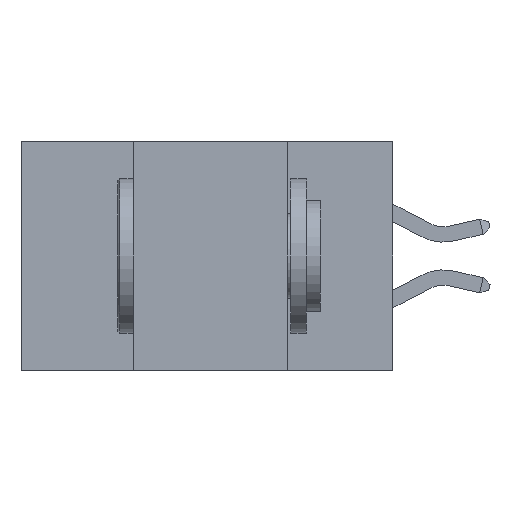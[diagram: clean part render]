
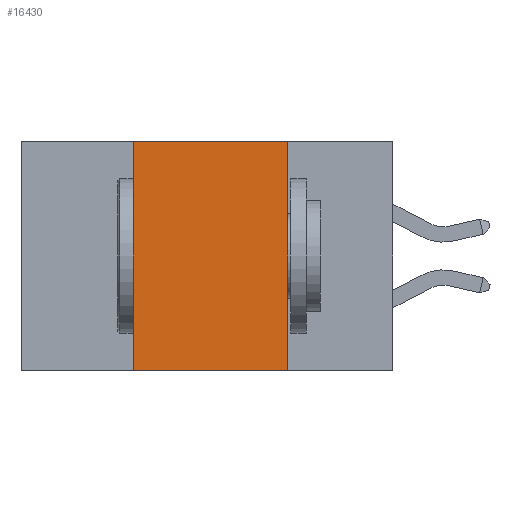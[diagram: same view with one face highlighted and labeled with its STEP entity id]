
A CAD part, left-side view. The second image highlights one B-rep face of the part: STEP entity #16430.
In plain terms, the highlighted planar face has unit normal (-1, 0, 0).
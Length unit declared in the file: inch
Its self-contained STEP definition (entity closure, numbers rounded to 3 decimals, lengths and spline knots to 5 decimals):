
#377 = VERTEX_POINT ( 'NONE', #13015 ) ;
#747 = VECTOR ( 'NONE', #12269, 39.37008 ) ;
#751 = EDGE_CURVE ( 'NONE', #3571, #23676, #10433, .T. ) ;
#1999 = FACE_OUTER_BOUND ( 'NONE', #18208, .T. ) ;
#2033 = CARTESIAN_POINT ( 'NONE',  ( 0., 0.17, 0. ) ) ;
#3480 = CARTESIAN_POINT ( 'NONE',  ( 0., 0.42, 0. ) ) ;
#3571 = VERTEX_POINT ( 'NONE', #21152 ) ;
#5234 = LINE ( 'NONE', #22747, #747 ) ;
#5465 = EDGE_CURVE ( 'NONE', #15761, #377, #5234, .T. ) ;
#5476 = PLANE ( 'NONE',  #8783 ) ;
#5738 = LINE ( 'NONE', #25685, #24884 ) ;
#5757 = DIRECTION ( 'NONE',  ( 0., 0., 1. ) ) ;
#6698 = LINE ( 'NONE', #3480, #24538 ) ;
#7764 = CARTESIAN_POINT ( 'NONE',  ( 0., 0.6, 0. ) ) ;
#8783 = AXIS2_PLACEMENT_3D ( 'NONE', #7764, #26142, #13625 ) ;
#10433 = LINE ( 'NONE', #17505, #19485 ) ;
#11803 = ORIENTED_EDGE ( 'NONE', *, *, #5465, .T. ) ;
#12073 = ORIENTED_EDGE ( 'NONE', *, *, #18575, .F. ) ;
#12269 = DIRECTION ( 'NONE',  ( 0., -1., 0. ) ) ;
#13015 = CARTESIAN_POINT ( 'NONE',  ( 0., 0.17, -0.37 ) ) ;
#13625 = DIRECTION ( 'NONE',  ( 0., 0., -1. ) ) ;
#13875 = ORIENTED_EDGE ( 'NONE', *, *, #18766, .F. ) ;
#15761 = VERTEX_POINT ( 'NONE', #23982 ) ;
#16430 = ADVANCED_FACE ( 'NONE', ( #1999 ), #5476, .F. ) ;
#17505 = CARTESIAN_POINT ( 'NONE',  ( 0., 0.6, 0. ) ) ;
#17787 = DIRECTION ( 'NONE',  ( 0., 0., -1. ) ) ;
#18208 = EDGE_LOOP ( 'NONE', ( #12073, #26581, #13875, #11803 ) ) ;
#18575 = EDGE_CURVE ( 'NONE', #23676, #377, #5738, .T. ) ;
#18766 = EDGE_CURVE ( 'NONE', #15761, #3571, #6698, .T. ) ;
#19485 = VECTOR ( 'NONE', #21606, 39.37008 ) ;
#21152 = CARTESIAN_POINT ( 'NONE',  ( 0., 0.42, 0. ) ) ;
#21606 = DIRECTION ( 'NONE',  ( 0., -1., 0. ) ) ;
#22747 = CARTESIAN_POINT ( 'NONE',  ( 0., 0.6, -0.37 ) ) ;
#23676 = VERTEX_POINT ( 'NONE', #2033 ) ;
#23982 = CARTESIAN_POINT ( 'NONE',  ( 0., 0.42, -0.37 ) ) ;
#24538 = VECTOR ( 'NONE', #5757, 39.37008 ) ;
#24884 = VECTOR ( 'NONE', #17787, 39.37008 ) ;
#25685 = CARTESIAN_POINT ( 'NONE',  ( 0., 0.17, 0. ) ) ;
#26142 = DIRECTION ( 'NONE',  ( 1., 0., 0. ) ) ;
#26581 = ORIENTED_EDGE ( 'NONE', *, *, #751, .F. ) ;
